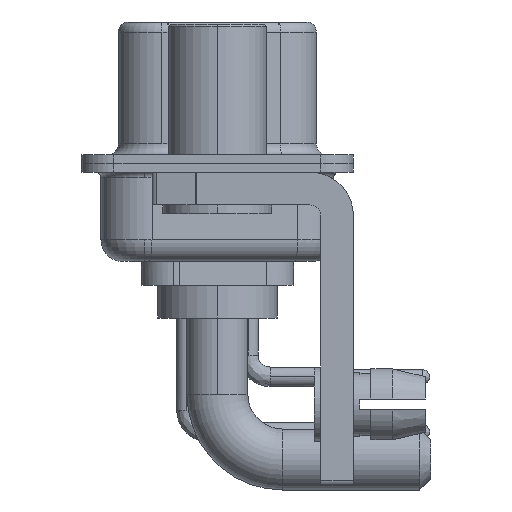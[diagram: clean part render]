
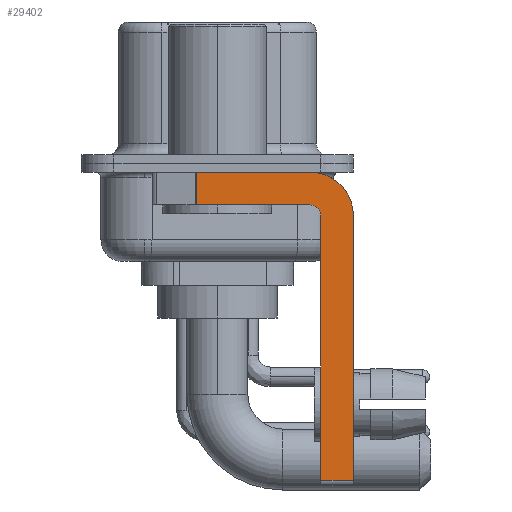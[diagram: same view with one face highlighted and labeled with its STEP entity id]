
A CAD part, left-side view. The second image highlights one B-rep face of the part: STEP entity #29402.
In plain terms, the highlighted planar face has unit normal (-1, 0, 0).
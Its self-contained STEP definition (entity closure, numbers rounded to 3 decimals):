
#267 = DIRECTION ( 'NONE',  ( 1., 0., 0. ) ) ;
#1295 = VERTEX_POINT ( 'NONE', #9757 ) ;
#1572 = VECTOR ( 'NONE', #4086, 1000. ) ;
#2039 = EDGE_CURVE ( 'NONE', #1295, #5314, #20333, .T. ) ;
#2592 = AXIS2_PLACEMENT_3D ( 'NONE', #10285, #267, #19526 ) ;
#2624 = DIRECTION ( 'NONE',  ( 0., 1., 0. ) ) ;
#2646 = VERTEX_POINT ( 'NONE', #6531 ) ;
#2809 = LINE ( 'NONE', #17540, #28577 ) ;
#3715 = ORIENTED_EDGE ( 'NONE', *, *, #2039, .T. ) ;
#3891 = VERTEX_POINT ( 'NONE', #5357 ) ;
#4086 = DIRECTION ( 'NONE',  ( 0., 0., -1. ) ) ;
#5111 = PLANE ( 'NONE',  #2592 ) ;
#5314 = VERTEX_POINT ( 'NONE', #6777 ) ;
#5357 = CARTESIAN_POINT ( 'NONE',  ( -2.9, -6.25, -14.55 ) ) ;
#5397 = CARTESIAN_POINT ( 'NONE',  ( -2.9, -4.25, -0.4 ) ) ;
#5511 = EDGE_CURVE ( 'NONE', #22528, #5685, #6938, .T. ) ;
#5685 = VERTEX_POINT ( 'NONE', #10773 ) ;
#5721 = VERTEX_POINT ( 'NONE', #26108 ) ;
#6449 = LINE ( 'NONE', #23355, #1572 ) ;
#6506 = VECTOR ( 'NONE', #21105, 1000. ) ;
#6531 = CARTESIAN_POINT ( 'NONE',  ( -2.9, -6.25, -2.4 ) ) ;
#6544 = CIRCLE ( 'NONE', #17042, 0.5 ) ;
#6777 = CARTESIAN_POINT ( 'NONE',  ( -2.9, 0.978, -1.9 ) ) ;
#6938 = LINE ( 'NONE', #16483, #24885 ) ;
#7932 = CARTESIAN_POINT ( 'NONE',  ( -2.9, -4.75, -14.55 ) ) ;
#7981 = EDGE_CURVE ( 'NONE', #11131, #2646, #23575, .T. ) ;
#9609 = EDGE_CURVE ( 'NONE', #2646, #3891, #6449, .T. ) ;
#9697 = ORIENTED_EDGE ( 'NONE', *, *, #27796, .F. ) ;
#9757 = CARTESIAN_POINT ( 'NONE',  ( -2.9, 0.978, -0.4 ) ) ;
#9906 = EDGE_CURVE ( 'NONE', #22528, #3891, #2809, .T. ) ;
#10285 = CARTESIAN_POINT ( 'NONE',  ( -2.9, -4.25, -2.4 ) ) ;
#10597 = VECTOR ( 'NONE', #2624, 1000. ) ;
#10607 = DIRECTION ( 'NONE',  ( 0., 0., -1. ) ) ;
#10773 = CARTESIAN_POINT ( 'NONE',  ( -2.9, -4.75, -2.4 ) ) ;
#11131 = VERTEX_POINT ( 'NONE', #5397 ) ;
#12166 = ORIENTED_EDGE ( 'NONE', *, *, #5511, .F. ) ;
#12567 = AXIS2_PLACEMENT_3D ( 'NONE', #12949, #22489, #10607 ) ;
#12949 = CARTESIAN_POINT ( 'NONE',  ( -2.9, -4.25, -2.4 ) ) ;
#13159 = CARTESIAN_POINT ( 'NONE',  ( -2.9, -4.25, -2.4 ) ) ;
#14140 = DIRECTION ( 'NONE',  ( 0., 0., 1. ) ) ;
#14212 = CARTESIAN_POINT ( 'NONE',  ( -2.9, 3., -0.4 ) ) ;
#15030 = DIRECTION ( 'NONE',  ( -1., 0., 0. ) ) ;
#15781 = CARTESIAN_POINT ( 'NONE',  ( -2.9, 0.978, -1.9 ) ) ;
#16483 = CARTESIAN_POINT ( 'NONE',  ( -2.9, -4.75, -14.8 ) ) ;
#16877 = LINE ( 'NONE', #28743, #10597 ) ;
#17042 = AXIS2_PLACEMENT_3D ( 'NONE', #13159, #15030, #20189 ) ;
#17540 = CARTESIAN_POINT ( 'NONE',  ( -2.9, -4.25, -14.55 ) ) ;
#19526 = DIRECTION ( 'NONE',  ( 0., 0., -1. ) ) ;
#19656 = EDGE_CURVE ( 'NONE', #5685, #5721, #6544, .T. ) ;
#20189 = DIRECTION ( 'NONE',  ( 0., 0., 1. ) ) ;
#20296 = ORIENTED_EDGE ( 'NONE', *, *, #29384, .F. ) ;
#20333 = LINE ( 'NONE', #15781, #21314 ) ;
#21105 = DIRECTION ( 'NONE',  ( 0., -1., 0. ) ) ;
#21314 = VECTOR ( 'NONE', #27362, 1000. ) ;
#21714 = FACE_OUTER_BOUND ( 'NONE', #29333, .T. ) ;
#22489 = DIRECTION ( 'NONE',  ( 1., 0., 0. ) ) ;
#22528 = VERTEX_POINT ( 'NONE', #7932 ) ;
#23355 = CARTESIAN_POINT ( 'NONE',  ( -2.9, -6.25, -2.4 ) ) ;
#23575 = CIRCLE ( 'NONE', #12567, 2. ) ;
#23756 = ORIENTED_EDGE ( 'NONE', *, *, #19656, .F. ) ;
#24885 = VECTOR ( 'NONE', #14140, 1000. ) ;
#26108 = CARTESIAN_POINT ( 'NONE',  ( -2.9, -4.25, -1.9 ) ) ;
#26467 = ORIENTED_EDGE ( 'NONE', *, *, #9906, .T. ) ;
#27069 = DIRECTION ( 'NONE',  ( 0., -1., 0. ) ) ;
#27362 = DIRECTION ( 'NONE',  ( 0., 0., -1. ) ) ;
#27796 = EDGE_CURVE ( 'NONE', #1295, #11131, #30453, .T. ) ;
#28577 = VECTOR ( 'NONE', #27069, 1000. ) ;
#28743 = CARTESIAN_POINT ( 'NONE',  ( -2.9, -4.25, -1.9 ) ) ;
#29333 = EDGE_LOOP ( 'NONE', ( #9697, #3715, #20296, #23756, #12166, #26467, #30821, #30344 ) ) ;
#29384 = EDGE_CURVE ( 'NONE', #5721, #5314, #16877, .T. ) ;
#29402 = ADVANCED_FACE ( 'NONE', ( #21714 ), #5111, .F. ) ;
#30344 = ORIENTED_EDGE ( 'NONE', *, *, #7981, .F. ) ;
#30453 = LINE ( 'NONE', #14212, #6506 ) ;
#30821 = ORIENTED_EDGE ( 'NONE', *, *, #9609, .F. ) ;
